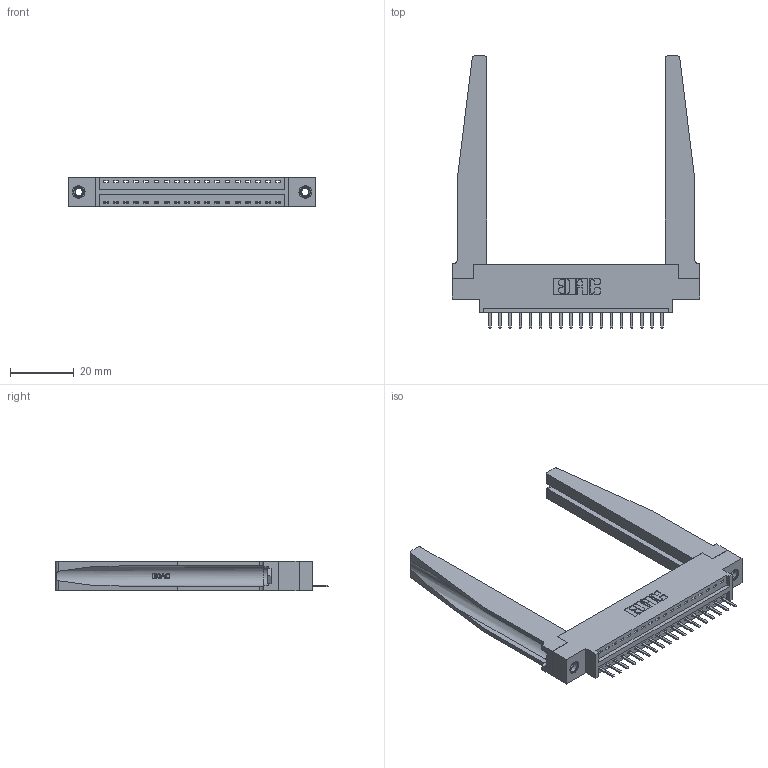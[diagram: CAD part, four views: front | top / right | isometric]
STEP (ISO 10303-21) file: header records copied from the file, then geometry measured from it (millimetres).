
FILE_DESCRIPTION (( 'STEP AP203' ), '1' );
FILE_NAME ('346-018-520-678.STEP', '2022-05-05T13:52:24', ( '' ), ( '' ), 'SwSTEP 2.0', 'SolidWorks 2020', '' );
FILE_SCHEMA (( 'CONFIG_CONTROL_DESIGN' ));
Length unit declared in the file: inch
Products named in the file (5): 345-292-001_345-293-120; 346 Part_0.170 Offset - 0.156 Dia-TH; 346-018-520-678; 346-220-078_345-220-078; 345-250-001_345-250-001-102
Assembly tree (23 placements, depth 2):
  346-018-520-678
    346 Part_0.170 Offset - 0.156 Dia-TH
    345-292-001_345-293-120  x18
    346-220-078_345-220-078  x2
    345-250-001_345-250-001-102  x2
Bounding box: 77.72 x 85.29 x 9.4 mm (x, y, z)
Volume: 13958.9 mm3; surface area: 15112.6 mm2
Topology: 23 solids, 23 shells, 1490 faces, 4297 edges, 2806 vertices
Faces by surface type: plane 992, cylinder 446, bspline 36, cone 12, torus 4
Entity records: 19812 total; most frequent: CARTESIAN_POINT 4331, ORIENTED_EDGE 3158, DIRECTION 2821, EDGE_CURVE 1579, LINE 1277, VECTOR 1277, VERTEX_POINT 1044, AXIS2_PLACEMENT_3D 772
